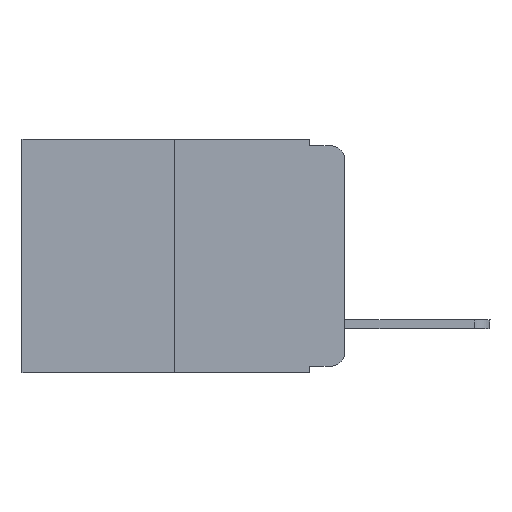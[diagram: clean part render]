
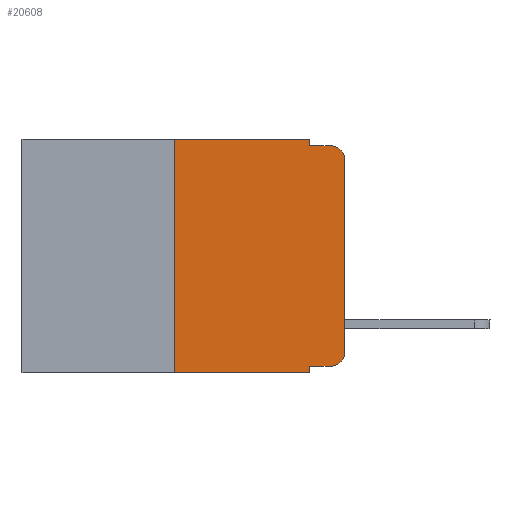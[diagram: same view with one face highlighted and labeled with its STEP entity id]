
A CAD part, left-side view. The second image highlights one B-rep face of the part: STEP entity #20608.
In plain terms, the highlighted planar face has unit normal (-1, 0, 0).
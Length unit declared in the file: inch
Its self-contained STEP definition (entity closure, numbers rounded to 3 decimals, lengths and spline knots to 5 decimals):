
#156 = EDGE_CURVE ( 'NONE', #13880, #2868, #5194, .T. ) ;
#319 = DIRECTION ( 'NONE',  ( 0., 0., -1. ) ) ;
#452 = CARTESIAN_POINT ( 'NONE',  ( 0., 0.02, -0.333 ) ) ;
#741 = CIRCLE ( 'NONE', #17358, 0.02 ) ;
#971 = ORIENTED_EDGE ( 'NONE', *, *, #7067, .T. ) ;
#1174 = VERTEX_POINT ( 'NONE', #17447 ) ;
#1239 = VECTOR ( 'NONE', #319, 39.37008 ) ;
#1315 = EDGE_CURVE ( 'NONE', #8855, #11489, #8616, .T. ) ;
#1732 = DIRECTION ( 'NONE',  ( 0., 0., 1. ) ) ;
#1933 = CARTESIAN_POINT ( 'NONE',  ( 0., 0.02, -0.01 ) ) ;
#2868 = VERTEX_POINT ( 'NONE', #1933 ) ;
#3278 = VERTEX_POINT ( 'NONE', #452 ) ;
#3664 = CARTESIAN_POINT ( 'NONE',  ( 0., 0.02, -0.313 ) ) ;
#3706 = CARTESIAN_POINT ( 'NONE',  ( 0., 0.25, 0. ) ) ;
#3993 = DIRECTION ( 'NONE',  ( -1., 0., 0. ) ) ;
#4363 = EDGE_CURVE ( 'NONE', #19665, #9969, #21881, .T. ) ;
#4624 = VECTOR ( 'NONE', #12053, 39.37008 ) ;
#5194 = CIRCLE ( 'NONE', #22588, 0.02 ) ;
#5363 = LINE ( 'NONE', #12734, #8807 ) ;
#5946 = ORIENTED_EDGE ( 'NONE', *, *, #10638, .F. ) ;
#6513 = CARTESIAN_POINT ( 'NONE',  ( 0., 0., -0.03 ) ) ;
#6577 = VERTEX_POINT ( 'NONE', #14585 ) ;
#7062 = ORIENTED_EDGE ( 'NONE', *, *, #14136, .F. ) ;
#7067 = EDGE_CURVE ( 'NONE', #3278, #6577, #741, .T. ) ;
#7105 = CARTESIAN_POINT ( 'NONE',  ( 0., 0.051, -0.333 ) ) ;
#7134 = CARTESIAN_POINT ( 'NONE',  ( 0., 0.051, -0.333 ) ) ;
#7239 = CARTESIAN_POINT ( 'NONE',  ( 0., 0.473, 0. ) ) ;
#7292 = VECTOR ( 'NONE', #11077, 39.37008 ) ;
#7846 = CARTESIAN_POINT ( 'NONE',  ( 0., 0.051, -0.01 ) ) ;
#8616 = LINE ( 'NONE', #23485, #20700 ) ;
#8807 = VECTOR ( 'NONE', #1732, 39.37008 ) ;
#8855 = VERTEX_POINT ( 'NONE', #7134 ) ;
#8876 = DIRECTION ( 'NONE',  ( 0., 0., -1. ) ) ;
#8942 = DIRECTION ( 'NONE',  ( 0., -1., 0. ) ) ;
#8954 = ORIENTED_EDGE ( 'NONE', *, *, #17502, .T. ) ;
#9160 = DIRECTION ( 'NONE',  ( 1., 0., 0. ) ) ;
#9490 = DIRECTION ( 'NONE',  ( 0., -1., 0. ) ) ;
#9969 = VERTEX_POINT ( 'NONE', #11612 ) ;
#9999 = LINE ( 'NONE', #7846, #17721 ) ;
#10610 = LINE ( 'NONE', #7105, #4624 ) ;
#10638 = EDGE_CURVE ( 'NONE', #9969, #1174, #22354, .T. ) ;
#11002 = CARTESIAN_POINT ( 'NONE',  ( 0., 0.051, -0.343 ) ) ;
#11077 = DIRECTION ( 'NONE',  ( 0., 0., 1. ) ) ;
#11142 = EDGE_CURVE ( 'NONE', #21528, #11489, #21956, .T. ) ;
#11462 = DIRECTION ( 'NONE',  ( 0., 0., -1. ) ) ;
#11489 = VERTEX_POINT ( 'NONE', #11002 ) ;
#11612 = CARTESIAN_POINT ( 'NONE',  ( 0., 0.051, 0. ) ) ;
#12053 = DIRECTION ( 'NONE',  ( 0., -1., 0. ) ) ;
#12544 = PLANE ( 'NONE',  #13974 ) ;
#12734 = CARTESIAN_POINT ( 'NONE',  ( 0., 0., 0. ) ) ;
#13006 = ORIENTED_EDGE ( 'NONE', *, *, #1315, .F. ) ;
#13297 = CARTESIAN_POINT ( 'NONE',  ( 0., 0.02, -0.03 ) ) ;
#13320 = EDGE_CURVE ( 'NONE', #6577, #13880, #5363, .T. ) ;
#13518 = EDGE_LOOP ( 'NONE', ( #14817, #23106, #22070, #5946, #17425, #7062, #18339, #13006, #8954, #971 ) ) ;
#13759 = EDGE_CURVE ( 'NONE', #1174, #2868, #9999, .T. ) ;
#13880 = VERTEX_POINT ( 'NONE', #6513 ) ;
#13974 = AXIS2_PLACEMENT_3D ( 'NONE', #18354, #9160, #17429 ) ;
#14136 = EDGE_CURVE ( 'NONE', #21528, #19665, #20285, .T. ) ;
#14309 = CARTESIAN_POINT ( 'NONE',  ( 0., 0.25, 0. ) ) ;
#14377 = VECTOR ( 'NONE', #9490, 39.37008 ) ;
#14539 = CARTESIAN_POINT ( 'NONE',  ( 0., 0.25, -0.343 ) ) ;
#14585 = CARTESIAN_POINT ( 'NONE',  ( 0., 0., -0.313 ) ) ;
#14817 = ORIENTED_EDGE ( 'NONE', *, *, #13320, .T. ) ;
#17358 = AXIS2_PLACEMENT_3D ( 'NONE', #3664, #18421, #8876 ) ;
#17396 = DIRECTION ( 'NONE',  ( 0., -1., 0. ) ) ;
#17425 = ORIENTED_EDGE ( 'NONE', *, *, #4363, .F. ) ;
#17429 = DIRECTION ( 'NONE',  ( 0., 0., -1. ) ) ;
#17447 = CARTESIAN_POINT ( 'NONE',  ( 0., 0.051, -0.01 ) ) ;
#17502 = EDGE_CURVE ( 'NONE', #8855, #3278, #10610, .T. ) ;
#17721 = VECTOR ( 'NONE', #17396, 39.37008 ) ;
#18244 = CARTESIAN_POINT ( 'NONE',  ( 0., 0.051, 0. ) ) ;
#18281 = VECTOR ( 'NONE', #8942, 39.37008 ) ;
#18339 = ORIENTED_EDGE ( 'NONE', *, *, #11142, .T. ) ;
#18354 = CARTESIAN_POINT ( 'NONE',  ( 0., 0.473, 0. ) ) ;
#18421 = DIRECTION ( 'NONE',  ( -1., 0., 0. ) ) ;
#19665 = VERTEX_POINT ( 'NONE', #14309 ) ;
#20285 = LINE ( 'NONE', #3706, #7292 ) ;
#20608 = ADVANCED_FACE ( 'NONE', ( #21980 ), #12544, .F. ) ;
#20700 = VECTOR ( 'NONE', #22020, 39.37008 ) ;
#21528 = VERTEX_POINT ( 'NONE', #14539 ) ;
#21881 = LINE ( 'NONE', #7239, #18281 ) ;
#21956 = LINE ( 'NONE', #22085, #14377 ) ;
#21980 = FACE_OUTER_BOUND ( 'NONE', #13518, .T. ) ;
#22020 = DIRECTION ( 'NONE',  ( 0., 0., -1. ) ) ;
#22070 = ORIENTED_EDGE ( 'NONE', *, *, #13759, .F. ) ;
#22085 = CARTESIAN_POINT ( 'NONE',  ( 0., 0.473, -0.343 ) ) ;
#22354 = LINE ( 'NONE', #18244, #1239 ) ;
#22588 = AXIS2_PLACEMENT_3D ( 'NONE', #13297, #3993, #11462 ) ;
#23106 = ORIENTED_EDGE ( 'NONE', *, *, #156, .T. ) ;
#23485 = CARTESIAN_POINT ( 'NONE',  ( 0., 0.051, 0. ) ) ;
